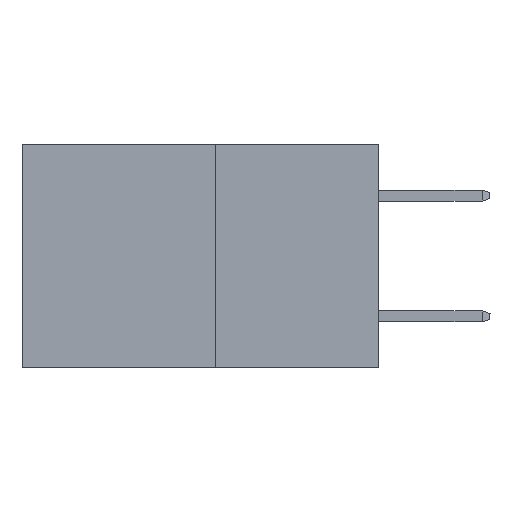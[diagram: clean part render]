
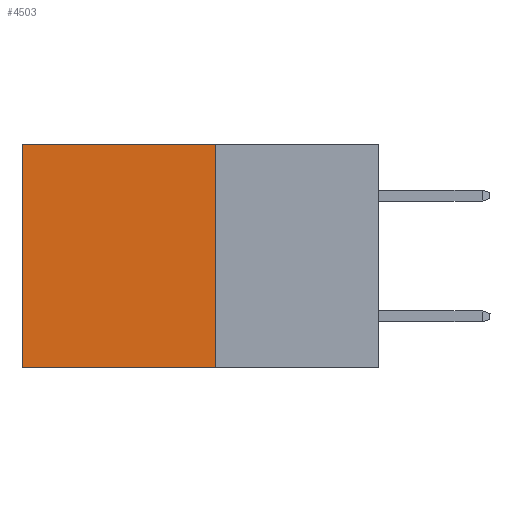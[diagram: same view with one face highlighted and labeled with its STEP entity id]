
A CAD part, left-side view. The second image highlights one B-rep face of the part: STEP entity #4503.
In plain terms, the highlighted planar face has unit normal (-1, 0, 0).
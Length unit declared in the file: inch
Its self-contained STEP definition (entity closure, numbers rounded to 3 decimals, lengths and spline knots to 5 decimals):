
#125 = EDGE_CURVE ( 'NONE', #8055, #221, #9329, .T. ) ;
#221 = VERTEX_POINT ( 'NONE', #6849 ) ;
#320 = EDGE_CURVE ( 'NONE', #221, #9271, #6177, .T. ) ;
#523 = DIRECTION ( 'NONE',  ( 0., 0., -1. ) ) ;
#540 = DIRECTION ( 'NONE',  ( 0., 1., 0. ) ) ;
#1722 = CARTESIAN_POINT ( 'NONE',  ( 0.277, 0.27, -0.37 ) ) ;
#2192 = DIRECTION ( 'NONE',  ( 0., 0., -1. ) ) ;
#2197 = ORIENTED_EDGE ( 'NONE', *, *, #320, .T. ) ;
#2691 = VECTOR ( 'NONE', #523, 39.37008 ) ;
#2973 = CARTESIAN_POINT ( 'NONE',  ( 0.277, 0.59, -0.37 ) ) ;
#2989 = CARTESIAN_POINT ( 'NONE',  ( 0.277, 0.27, 0. ) ) ;
#3007 = CARTESIAN_POINT ( 'NONE',  ( 0.277, 0.27, -0.37 ) ) ;
#3470 = CARTESIAN_POINT ( 'NONE',  ( 0.277, 0.27, -0.37 ) ) ;
#3694 = EDGE_CURVE ( 'NONE', #5777, #9271, #5714, .T. ) ;
#3980 = ORIENTED_EDGE ( 'NONE', *, *, #125, .T. ) ;
#4361 = VECTOR ( 'NONE', #2192, 39.37008 ) ;
#4503 = ADVANCED_FACE ( 'NONE', ( #10108 ), #7225, .F. ) ;
#4600 = AXIS2_PLACEMENT_3D ( 'NONE', #3470, #4747, #8099 ) ;
#4698 = ORIENTED_EDGE ( 'NONE', *, *, #6205, .F. ) ;
#4747 = DIRECTION ( 'NONE',  ( 1., 0., 0. ) ) ;
#5157 = CARTESIAN_POINT ( 'NONE',  ( 0.277, 0.59, -0.37 ) ) ;
#5714 = LINE ( 'NONE', #6899, #9431 ) ;
#5777 = VERTEX_POINT ( 'NONE', #1722 ) ;
#6100 = EDGE_LOOP ( 'NONE', ( #2197, #10300, #4698, #3980 ) ) ;
#6177 = LINE ( 'NONE', #5157, #4361 ) ;
#6205 = EDGE_CURVE ( 'NONE', #8055, #5777, #8583, .T. ) ;
#6849 = CARTESIAN_POINT ( 'NONE',  ( 0.277, 0.59, 0. ) ) ;
#6899 = CARTESIAN_POINT ( 'NONE',  ( 0.277, 0.27, -0.37 ) ) ;
#6906 = DIRECTION ( 'NONE',  ( 0., 1., 0. ) ) ;
#7225 = PLANE ( 'NONE',  #4600 ) ;
#8055 = VERTEX_POINT ( 'NONE', #9387 ) ;
#8099 = DIRECTION ( 'NONE',  ( 0., 0., -1. ) ) ;
#8583 = LINE ( 'NONE', #3007, #2691 ) ;
#9092 = VECTOR ( 'NONE', #540, 39.37008 ) ;
#9271 = VERTEX_POINT ( 'NONE', #2973 ) ;
#9329 = LINE ( 'NONE', #2989, #9092 ) ;
#9387 = CARTESIAN_POINT ( 'NONE',  ( 0.277, 0.27, 0. ) ) ;
#9431 = VECTOR ( 'NONE', #6906, 39.37008 ) ;
#10108 = FACE_OUTER_BOUND ( 'NONE', #6100, .T. ) ;
#10300 = ORIENTED_EDGE ( 'NONE', *, *, #3694, .F. ) ;
